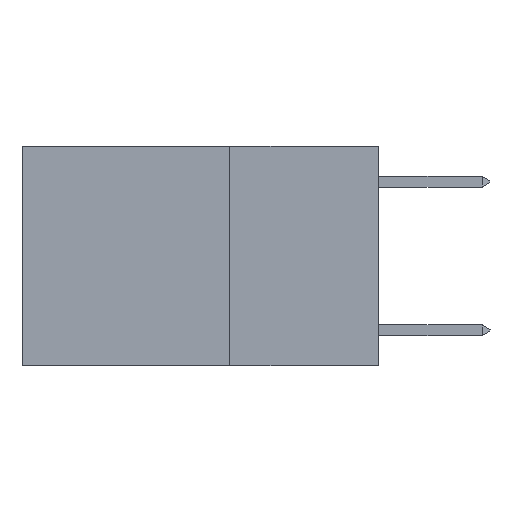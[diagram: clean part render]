
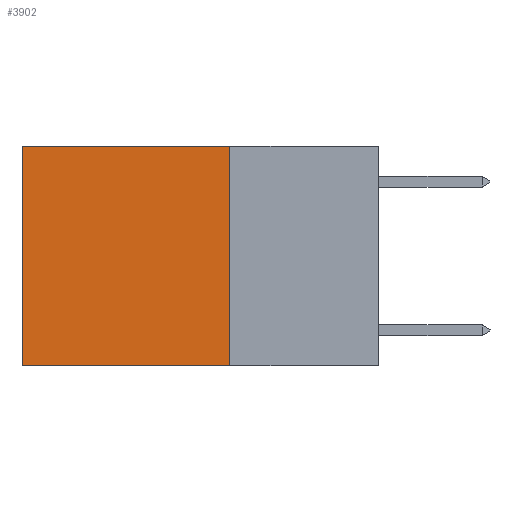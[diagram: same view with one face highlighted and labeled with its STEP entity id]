
A CAD part, left-side view. The second image highlights one B-rep face of the part: STEP entity #3902.
In plain terms, the highlighted planar face has unit normal (-1, 0, 0).
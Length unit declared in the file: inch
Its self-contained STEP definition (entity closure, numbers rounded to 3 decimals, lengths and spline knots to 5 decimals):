
#665 = CARTESIAN_POINT ( 'NONE',  ( 0.2625, 0.25, 0. ) ) ;
#750 = DIRECTION ( 'NONE',  ( 1., 0., 0. ) ) ;
#1583 = CARTESIAN_POINT ( 'NONE',  ( 0.2625, 0.6, 0. ) ) ;
#1769 = ORIENTED_EDGE ( 'NONE', *, *, #13142, .T. ) ;
#1809 = CARTESIAN_POINT ( 'NONE',  ( 0.2625, 0.6, 0. ) ) ;
#2076 = CARTESIAN_POINT ( 'NONE',  ( 0.2625, 0.25, 0. ) ) ;
#2239 = EDGE_CURVE ( 'NONE', #25060, #17731, #24025, .T. ) ;
#2277 = FACE_OUTER_BOUND ( 'NONE', #7649, .T. ) ;
#2813 = CARTESIAN_POINT ( 'NONE',  ( 0.2625, 0.25, 0. ) ) ;
#3902 = ADVANCED_FACE ( 'NONE', ( #2277 ), #21561, .F. ) ;
#5039 = DIRECTION ( 'NONE',  ( 0., 1., 0. ) ) ;
#5719 = CARTESIAN_POINT ( 'NONE',  ( 0.2625, 0.6, -0.37 ) ) ;
#5732 = ORIENTED_EDGE ( 'NONE', *, *, #7896, .T. ) ;
#5899 = VECTOR ( 'NONE', #10485, 39.37008 ) ;
#6691 = ORIENTED_EDGE ( 'NONE', *, *, #20189, .F. ) ;
#6932 = CARTESIAN_POINT ( 'NONE',  ( 0.2625, 0.25, -0.37 ) ) ;
#7649 = EDGE_LOOP ( 'NONE', ( #1769, #11263, #6691, #5732 ) ) ;
#7778 = VERTEX_POINT ( 'NONE', #1809 ) ;
#7896 = EDGE_CURVE ( 'NONE', #14965, #7778, #20943, .T. ) ;
#8347 = LINE ( 'NONE', #1583, #12161 ) ;
#8628 = DIRECTION ( 'NONE',  ( 0., 0., -1. ) ) ;
#8909 = CARTESIAN_POINT ( 'NONE',  ( 0.2625, 0.25, -0.37 ) ) ;
#10485 = DIRECTION ( 'NONE',  ( 0., 1., 0. ) ) ;
#11263 = ORIENTED_EDGE ( 'NONE', *, *, #2239, .F. ) ;
#11392 = LINE ( 'NONE', #665, #21617 ) ;
#12161 = VECTOR ( 'NONE', #24987, 39.37008 ) ;
#13142 = EDGE_CURVE ( 'NONE', #7778, #17731, #8347, .T. ) ;
#13318 = DIRECTION ( 'NONE',  ( 0., 0., -1. ) ) ;
#14965 = VERTEX_POINT ( 'NONE', #16689 ) ;
#16594 = VECTOR ( 'NONE', #5039, 39.37008 ) ;
#16689 = CARTESIAN_POINT ( 'NONE',  ( 0.2625, 0.25, 0. ) ) ;
#17731 = VERTEX_POINT ( 'NONE', #5719 ) ;
#20189 = EDGE_CURVE ( 'NONE', #14965, #25060, #11392, .T. ) ;
#20943 = LINE ( 'NONE', #2076, #5899 ) ;
#21561 = PLANE ( 'NONE',  #27153 ) ;
#21617 = VECTOR ( 'NONE', #13318, 39.37008 ) ;
#24025 = LINE ( 'NONE', #8909, #16594 ) ;
#24987 = DIRECTION ( 'NONE',  ( 0., 0., -1. ) ) ;
#25060 = VERTEX_POINT ( 'NONE', #6932 ) ;
#27153 = AXIS2_PLACEMENT_3D ( 'NONE', #2813, #750, #8628 ) ;
